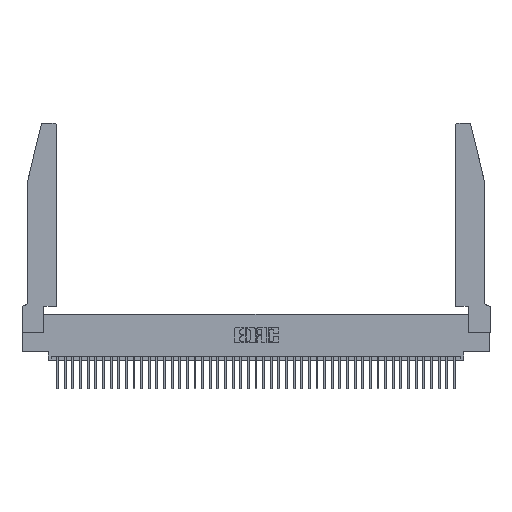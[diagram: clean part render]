
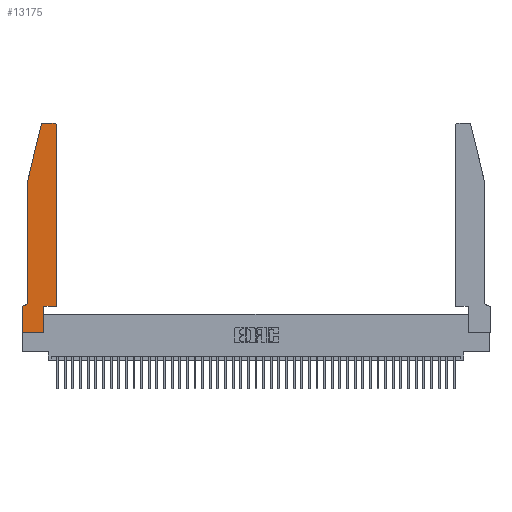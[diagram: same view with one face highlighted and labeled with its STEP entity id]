
A CAD part, top view. The second image highlights one B-rep face of the part: STEP entity #13175.
In plain terms, the highlighted planar face has unit normal (0, 0, 1).
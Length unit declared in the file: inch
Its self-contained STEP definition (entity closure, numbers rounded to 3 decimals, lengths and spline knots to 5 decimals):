
#251 = ORIENTED_EDGE ( 'NONE', *, *, #38963, .T. ) ;
#3076 = DIRECTION ( 'NONE',  ( 0., 0., 1. ) ) ;
#3356 = VERTEX_POINT ( 'NONE', #17518 ) ;
#3813 = PLANE ( 'NONE',  #16499 ) ;
#4557 = LINE ( 'NONE', #16212, #12791 ) ;
#4780 = CIRCLE ( 'NONE', #7765, 0.03 ) ;
#4909 = CARTESIAN_POINT ( 'NONE',  ( 0.4505, 2.72, 0.37 ) ) ;
#5376 = VECTOR ( 'NONE', #18495, 39.37008 ) ;
#6215 = CARTESIAN_POINT ( 'NONE',  ( 0.4505, 0.35, 0.37 ) ) ;
#7765 = AXIS2_PLACEMENT_3D ( 'NONE', #33315, #12450, #36754 ) ;
#7894 = CARTESIAN_POINT ( 'NONE',  ( 0.2605, 2.75, 0.37 ) ) ;
#8120 = ORIENTED_EDGE ( 'NONE', *, *, #43828, .T. ) ;
#8659 = CARTESIAN_POINT ( 'NONE',  ( 0.0755, 2., 0.37 ) ) ;
#9702 = LINE ( 'NONE', #42821, #27170 ) ;
#10246 = VERTEX_POINT ( 'NONE', #42971 ) ;
#10572 = VERTEX_POINT ( 'NONE', #30844 ) ;
#10953 = ORIENTED_EDGE ( 'NONE', *, *, #42134, .T. ) ;
#10974 = ORIENTED_EDGE ( 'NONE', *, *, #44422, .T. ) ;
#11535 = VERTEX_POINT ( 'NONE', #32561 ) ;
#11665 = CARTESIAN_POINT ( 'NONE',  ( 0.4505, 0.35, 0.37 ) ) ;
#12088 = CIRCLE ( 'NONE', #27386, 0.03 ) ;
#12450 = DIRECTION ( 'NONE',  ( 0., 0., 1. ) ) ;
#12548 = LINE ( 'NONE', #25745, #31131 ) ;
#12791 = VECTOR ( 'NONE', #19592, 39.37008 ) ;
#12799 = ORIENTED_EDGE ( 'NONE', *, *, #16868, .T. ) ;
#13130 = VERTEX_POINT ( 'NONE', #28120 ) ;
#13175 = ADVANCED_FACE ( 'NONE', ( #38433 ), #3813, .T. ) ;
#13359 = DIRECTION ( 'NONE',  ( 0., 0., -1. ) ) ;
#13789 = CARTESIAN_POINT ( 'NONE',  ( 0.4205, 2.75, 0.37 ) ) ;
#14046 = LINE ( 'NONE', #11665, #31495 ) ;
#14401 = DIRECTION ( 'NONE',  ( 1., 0., 0. ) ) ;
#14571 = CARTESIAN_POINT ( 'NONE',  ( 0.2865, 0.35, 0.37 ) ) ;
#15012 = VERTEX_POINT ( 'NONE', #13789 ) ;
#15250 = LINE ( 'NONE', #15721, #42810 ) ;
#15378 = DIRECTION ( 'NONE',  ( 0., 1., 0. ) ) ;
#15721 = CARTESIAN_POINT ( 'NONE',  ( 0.4505, 0.35, 0.37 ) ) ;
#16067 = VECTOR ( 'NONE', #43729, 39.37008 ) ;
#16111 = DIRECTION ( 'NONE',  ( 0., 1., 0. ) ) ;
#16212 = CARTESIAN_POINT ( 'NONE',  ( 0.0755, 2., 0.37 ) ) ;
#16499 = AXIS2_PLACEMENT_3D ( 'NONE', #31771, #35210, #14401 ) ;
#16697 = EDGE_CURVE ( 'NONE', #10572, #23530, #4780, .T. ) ;
#16868 = EDGE_CURVE ( 'NONE', #13130, #11535, #43335, .T. ) ;
#17114 = ORIENTED_EDGE ( 'NONE', *, *, #40269, .T. ) ;
#17418 = EDGE_CURVE ( 'NONE', #10246, #20919, #23914, .T. ) ;
#17518 = CARTESIAN_POINT ( 'NONE',  ( 0., 0., 0.37 ) ) ;
#18483 = VERTEX_POINT ( 'NONE', #4909 ) ;
#18495 = DIRECTION ( 'NONE',  ( -1., 0., 0. ) ) ;
#19592 = DIRECTION ( 'NONE',  ( -0.239, -0.971, 0. ) ) ;
#19861 = EDGE_CURVE ( 'NONE', #30411, #13130, #24847, .T. ) ;
#20122 = EDGE_LOOP ( 'NONE', ( #31011, #20875, #17114, #22061, #12799, #10974, #38719, #32758, #21205, #8120, #251, #10953 ) ) ;
#20875 = ORIENTED_EDGE ( 'NONE', *, *, #16697, .T. ) ;
#20919 = VERTEX_POINT ( 'NONE', #14571 ) ;
#21205 = ORIENTED_EDGE ( 'NONE', *, *, #17418, .T. ) ;
#22061 = ORIENTED_EDGE ( 'NONE', *, *, #19861, .T. ) ;
#23530 = VERTEX_POINT ( 'NONE', #25542 ) ;
#23914 = LINE ( 'NONE', #43719, #32082 ) ;
#24056 = CARTESIAN_POINT ( 'NONE',  ( 0.4205, 2.72, 0.37 ) ) ;
#24847 = LINE ( 'NONE', #8659, #42063 ) ;
#25292 = EDGE_CURVE ( 'NONE', #3356, #10246, #26380, .T. ) ;
#25542 = CARTESIAN_POINT ( 'NONE',  ( 0.25487, 2.72718, 0.37 ) ) ;
#25599 = CARTESIAN_POINT ( 'NONE',  ( 0., 0.35, 0.37 ) ) ;
#25658 = DIRECTION ( 'NONE',  ( -1., 0., 0. ) ) ;
#25745 = CARTESIAN_POINT ( 'NONE',  ( 0., 0., 0.37 ) ) ;
#26179 = DIRECTION ( 'NONE',  ( 1., 0., 0. ) ) ;
#26290 = CARTESIAN_POINT ( 'NONE',  ( 0.0755, 2., 0.37 ) ) ;
#26380 = LINE ( 'NONE', #26591, #16067 ) ;
#26591 = CARTESIAN_POINT ( 'NONE',  ( 0., 0., 0.37 ) ) ;
#27170 = VECTOR ( 'NONE', #25658, 39.37008 ) ;
#27317 = VERTEX_POINT ( 'NONE', #6215 ) ;
#27386 = AXIS2_PLACEMENT_3D ( 'NONE', #24056, #3076, #27525 ) ;
#27525 = DIRECTION ( 'NONE',  ( 1., 0., 0. ) ) ;
#28120 = CARTESIAN_POINT ( 'NONE',  ( 0.0755, 0.42, 0.37 ) ) ;
#29277 = DIRECTION ( 'NONE',  ( 0., -1., 0. ) ) ;
#29565 = DIRECTION ( 'NONE',  ( 0., -1., 0. ) ) ;
#30411 = VERTEX_POINT ( 'NONE', #26290 ) ;
#30844 = CARTESIAN_POINT ( 'NONE',  ( 0.284, 2.75, 0.37 ) ) ;
#31011 = ORIENTED_EDGE ( 'NONE', *, *, #43664, .T. ) ;
#31131 = VECTOR ( 'NONE', #29277, 39.37008 ) ;
#31164 = AXIS2_PLACEMENT_3D ( 'NONE', #34197, #13359, #37628 ) ;
#31495 = VECTOR ( 'NONE', #15378, 39.37008 ) ;
#31771 = CARTESIAN_POINT ( 'NONE',  ( 0., 0.35, 0.37 ) ) ;
#32082 = VECTOR ( 'NONE', #16111, 39.37008 ) ;
#32561 = CARTESIAN_POINT ( 'NONE',  ( 0.0055, 0.35, 0.37 ) ) ;
#32758 = ORIENTED_EDGE ( 'NONE', *, *, #25292, .T. ) ;
#33315 = CARTESIAN_POINT ( 'NONE',  ( 0.284, 2.72, 0.37 ) ) ;
#34197 = CARTESIAN_POINT ( 'NONE',  ( 0.0055, 0.42, 0.37 ) ) ;
#35210 = DIRECTION ( 'NONE',  ( 0., 0., 1. ) ) ;
#36252 = VERTEX_POINT ( 'NONE', #25599 ) ;
#36261 = EDGE_CURVE ( 'NONE', #36252, #3356, #12548, .T. ) ;
#36754 = DIRECTION ( 'NONE',  ( 1., 0., 0. ) ) ;
#37628 = DIRECTION ( 'NONE',  ( -1., 0., 0. ) ) ;
#38433 = FACE_OUTER_BOUND ( 'NONE', #20122, .T. ) ;
#38719 = ORIENTED_EDGE ( 'NONE', *, *, #36261, .T. ) ;
#38963 = EDGE_CURVE ( 'NONE', #27317, #18483, #14046, .T. ) ;
#40269 = EDGE_CURVE ( 'NONE', #23530, #30411, #4557, .T. ) ;
#42063 = VECTOR ( 'NONE', #29565, 39.37008 ) ;
#42134 = EDGE_CURVE ( 'NONE', #18483, #15012, #12088, .T. ) ;
#42315 = LINE ( 'NONE', #7894, #5376 ) ;
#42810 = VECTOR ( 'NONE', #26179, 39.37008 ) ;
#42821 = CARTESIAN_POINT ( 'NONE',  ( 0.0755, 0.35, 0.37 ) ) ;
#42971 = CARTESIAN_POINT ( 'NONE',  ( 0.2865, 0., 0.37 ) ) ;
#43335 = CIRCLE ( 'NONE', #31164, 0.07 ) ;
#43664 = EDGE_CURVE ( 'NONE', #15012, #10572, #42315, .T. ) ;
#43719 = CARTESIAN_POINT ( 'NONE',  ( 0.2865, 0.35, 0.37 ) ) ;
#43729 = DIRECTION ( 'NONE',  ( 1., 0., 0. ) ) ;
#43828 = EDGE_CURVE ( 'NONE', #20919, #27317, #15250, .T. ) ;
#44422 = EDGE_CURVE ( 'NONE', #11535, #36252, #9702, .T. ) ;
